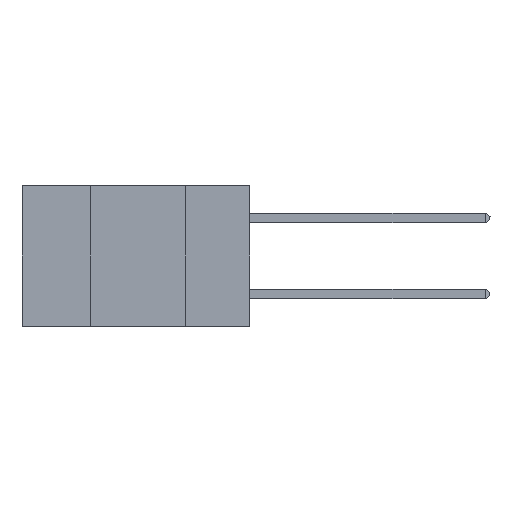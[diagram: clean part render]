
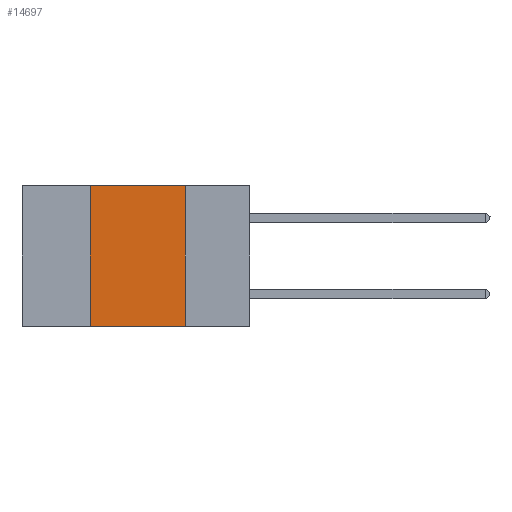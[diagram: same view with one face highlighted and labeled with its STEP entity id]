
A CAD part, left-side view. The second image highlights one B-rep face of the part: STEP entity #14697.
In plain terms, the highlighted planar face has unit normal (-1, 0, 0).
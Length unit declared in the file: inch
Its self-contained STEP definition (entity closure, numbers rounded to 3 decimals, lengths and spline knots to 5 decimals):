
#1007 = ORIENTED_EDGE ( 'NONE', *, *, #28177, .F. ) ;
#1664 = VERTEX_POINT ( 'NONE', #38979 ) ;
#2175 = VECTOR ( 'NONE', #31270, 39.37008 ) ;
#2517 = CARTESIAN_POINT ( 'NONE',  ( 0., 0.42, 0. ) ) ;
#2883 = DIRECTION ( 'NONE',  ( 1., 0., 0. ) ) ;
#3471 = CARTESIAN_POINT ( 'NONE',  ( 0., 0.6, -0.37 ) ) ;
#4872 = CARTESIAN_POINT ( 'NONE',  ( 0., 0.42, -0.37 ) ) ;
#7617 = VERTEX_POINT ( 'NONE', #4872 ) ;
#7653 = EDGE_CURVE ( 'NONE', #1664, #24464, #31306, .T. ) ;
#8283 = CARTESIAN_POINT ( 'NONE',  ( 0., 0.6, 0. ) ) ;
#10165 = EDGE_CURVE ( 'NONE', #16726, #1664, #36050, .T. ) ;
#11473 = LINE ( 'NONE', #2517, #22538 ) ;
#14319 = DIRECTION ( 'NONE',  ( 0., 0., 1. ) ) ;
#14697 = ADVANCED_FACE ( 'NONE', ( #27249 ), #24012, .F. ) ;
#15464 = VECTOR ( 'NONE', #29986, 39.37008 ) ;
#16726 = VERTEX_POINT ( 'NONE', #37918 ) ;
#22278 = ORIENTED_EDGE ( 'NONE', *, *, #7653, .F. ) ;
#22538 = VECTOR ( 'NONE', #14319, 39.37008 ) ;
#22992 = VECTOR ( 'NONE', #25841, 39.37008 ) ;
#24012 = PLANE ( 'NONE',  #31733 ) ;
#24464 = VERTEX_POINT ( 'NONE', #39612 ) ;
#25841 = DIRECTION ( 'NONE',  ( 0., 0., -1. ) ) ;
#27249 = FACE_OUTER_BOUND ( 'NONE', #36830, .T. ) ;
#28177 = EDGE_CURVE ( 'NONE', #7617, #16726, #11473, .T. ) ;
#29986 = DIRECTION ( 'NONE',  ( 0., -1., 0. ) ) ;
#31270 = DIRECTION ( 'NONE',  ( 0., -1., 0. ) ) ;
#31306 = LINE ( 'NONE', #31704, #22992 ) ;
#31704 = CARTESIAN_POINT ( 'NONE',  ( 0., 0.17, 0. ) ) ;
#31733 = AXIS2_PLACEMENT_3D ( 'NONE', #39786, #2883, #36542 ) ;
#34502 = LINE ( 'NONE', #3471, #2175 ) ;
#35240 = ORIENTED_EDGE ( 'NONE', *, *, #10165, .F. ) ;
#36050 = LINE ( 'NONE', #8283, #15464 ) ;
#36542 = DIRECTION ( 'NONE',  ( 0., 0., -1. ) ) ;
#36797 = ORIENTED_EDGE ( 'NONE', *, *, #39480, .T. ) ;
#36830 = EDGE_LOOP ( 'NONE', ( #22278, #35240, #1007, #36797 ) ) ;
#37918 = CARTESIAN_POINT ( 'NONE',  ( 0., 0.42, 0. ) ) ;
#38979 = CARTESIAN_POINT ( 'NONE',  ( 0., 0.17, 0. ) ) ;
#39480 = EDGE_CURVE ( 'NONE', #7617, #24464, #34502, .T. ) ;
#39612 = CARTESIAN_POINT ( 'NONE',  ( 0., 0.17, -0.37 ) ) ;
#39786 = CARTESIAN_POINT ( 'NONE',  ( 0., 0.6, 0. ) ) ;
